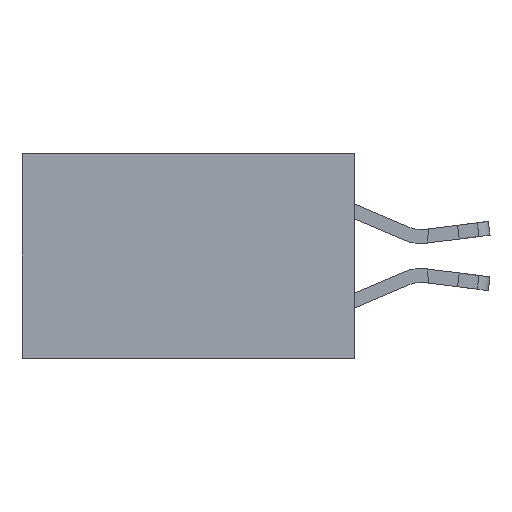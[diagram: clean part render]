
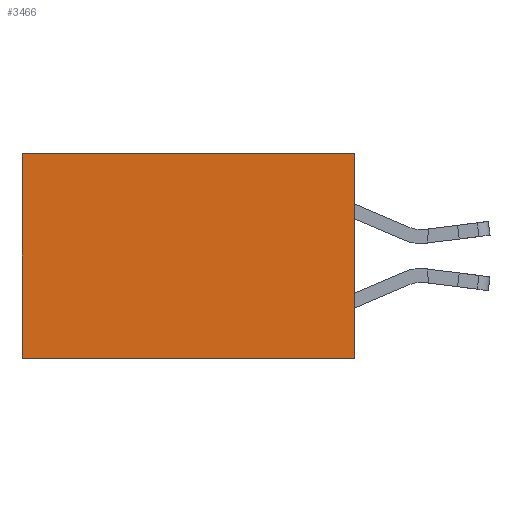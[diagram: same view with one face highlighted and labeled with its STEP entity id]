
A CAD part, left-side view. The second image highlights one B-rep face of the part: STEP entity #3466.
In plain terms, the highlighted planar face has unit normal (-1, 0, 0).
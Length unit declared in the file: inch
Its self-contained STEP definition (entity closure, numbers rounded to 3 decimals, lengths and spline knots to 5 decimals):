
#620 = DIRECTION ( 'NONE',  ( 0., 0., -1. ) ) ;
#1033 = ORIENTED_EDGE ( 'NONE', *, *, #8396, .F. ) ;
#2263 = EDGE_LOOP ( 'NONE', ( #15956, #1033, #5036, #11695 ) ) ;
#2969 = LINE ( 'NONE', #3195, #6323 ) ;
#3195 = CARTESIAN_POINT ( 'NONE',  ( 0.298, 0.6, 0. ) ) ;
#3466 = ADVANCED_FACE ( 'NONE', ( #9128 ), #14655, .F. ) ;
#3861 = VECTOR ( 'NONE', #16397, 39.37008 ) ;
#4544 = CARTESIAN_POINT ( 'NONE',  ( 0.298, 0., 0. ) ) ;
#4592 = CARTESIAN_POINT ( 'NONE',  ( 0.298, 0., 0. ) ) ;
#4945 = CARTESIAN_POINT ( 'NONE',  ( 0.298, 0., -0.37 ) ) ;
#5010 = CARTESIAN_POINT ( 'NONE',  ( 0.298, 0.6, -0.37 ) ) ;
#5036 = ORIENTED_EDGE ( 'NONE', *, *, #8666, .F. ) ;
#6323 = VECTOR ( 'NONE', #620, 39.37008 ) ;
#6943 = VERTEX_POINT ( 'NONE', #12126 ) ;
#7572 = LINE ( 'NONE', #4945, #3861 ) ;
#8396 = EDGE_CURVE ( 'NONE', #6943, #12041, #7572, .T. ) ;
#8666 = EDGE_CURVE ( 'NONE', #13170, #6943, #12565, .T. ) ;
#8688 = VECTOR ( 'NONE', #13387, 39.37008 ) ;
#9092 = LINE ( 'NONE', #4544, #8688 ) ;
#9128 = FACE_OUTER_BOUND ( 'NONE', #2263, .T. ) ;
#9159 = VECTOR ( 'NONE', #14129, 39.37008 ) ;
#10018 = CARTESIAN_POINT ( 'NONE',  ( 0.298, 0.6, 0. ) ) ;
#10465 = DIRECTION ( 'NONE',  ( 1., 0., 0. ) ) ;
#10912 = EDGE_CURVE ( 'NONE', #13170, #15380, #9092, .T. ) ;
#11534 = EDGE_CURVE ( 'NONE', #15380, #12041, #2969, .T. ) ;
#11695 = ORIENTED_EDGE ( 'NONE', *, *, #10912, .T. ) ;
#11729 = AXIS2_PLACEMENT_3D ( 'NONE', #13614, #10465, #16313 ) ;
#12041 = VERTEX_POINT ( 'NONE', #5010 ) ;
#12126 = CARTESIAN_POINT ( 'NONE',  ( 0.298, 0., -0.37 ) ) ;
#12565 = LINE ( 'NONE', #12863, #9159 ) ;
#12863 = CARTESIAN_POINT ( 'NONE',  ( 0.298, 0., 0. ) ) ;
#13170 = VERTEX_POINT ( 'NONE', #4592 ) ;
#13387 = DIRECTION ( 'NONE',  ( 0., 1., 0. ) ) ;
#13614 = CARTESIAN_POINT ( 'NONE',  ( 0.298, 0., 0. ) ) ;
#14129 = DIRECTION ( 'NONE',  ( 0., 0., -1. ) ) ;
#14655 = PLANE ( 'NONE',  #11729 ) ;
#15380 = VERTEX_POINT ( 'NONE', #10018 ) ;
#15956 = ORIENTED_EDGE ( 'NONE', *, *, #11534, .T. ) ;
#16313 = DIRECTION ( 'NONE',  ( 0., 0., -1. ) ) ;
#16397 = DIRECTION ( 'NONE',  ( 0., 1., 0. ) ) ;
